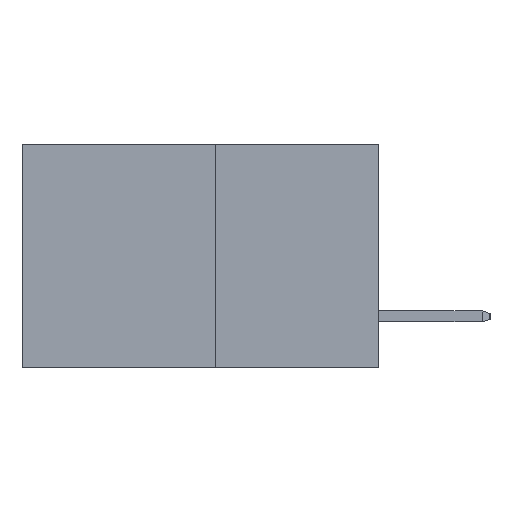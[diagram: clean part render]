
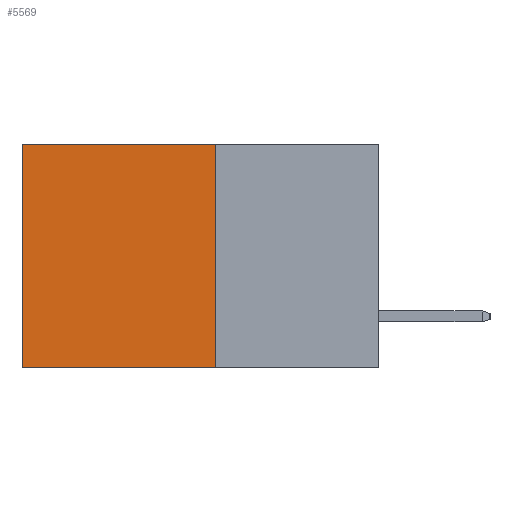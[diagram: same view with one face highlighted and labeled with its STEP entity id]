
A CAD part, left-side view. The second image highlights one B-rep face of the part: STEP entity #5569.
In plain terms, the highlighted planar face has unit normal (-1, 0, 0).
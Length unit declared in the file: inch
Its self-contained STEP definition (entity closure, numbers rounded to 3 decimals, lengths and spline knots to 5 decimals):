
#276 = CARTESIAN_POINT ( 'NONE',  ( 0.277, 0.27, -0.37 ) ) ;
#333 = VERTEX_POINT ( 'NONE', #5721 ) ;
#548 = VERTEX_POINT ( 'NONE', #2251 ) ;
#675 = ORIENTED_EDGE ( 'NONE', *, *, #3470, .F. ) ;
#1112 = DIRECTION ( 'NONE',  ( 1., 0., 0. ) ) ;
#1652 = CARTESIAN_POINT ( 'NONE',  ( 0.277, 0.59, -0.37 ) ) ;
#1995 = DIRECTION ( 'NONE',  ( 0., 1., 0. ) ) ;
#2251 = CARTESIAN_POINT ( 'NONE',  ( 0.277, 0.27, 0. ) ) ;
#2554 = LINE ( 'NONE', #5947, #4457 ) ;
#2792 = CARTESIAN_POINT ( 'NONE',  ( 0.277, 0.27, 0. ) ) ;
#3470 = EDGE_CURVE ( 'NONE', #8673, #333, #2554, .T. ) ;
#3576 = ORIENTED_EDGE ( 'NONE', *, *, #6366, .F. ) ;
#4077 = VECTOR ( 'NONE', #6676, 39.37008 ) ;
#4457 = VECTOR ( 'NONE', #6233, 39.37008 ) ;
#4651 = CARTESIAN_POINT ( 'NONE',  ( 0.277, 0.27, -0.37 ) ) ;
#4746 = AXIS2_PLACEMENT_3D ( 'NONE', #276, #1112, #6191 ) ;
#4806 = PLANE ( 'NONE',  #4746 ) ;
#4910 = EDGE_LOOP ( 'NONE', ( #8149, #675, #3576, #5305 ) ) ;
#4969 = LINE ( 'NONE', #7068, #5188 ) ;
#4987 = LINE ( 'NONE', #2792, #6616 ) ;
#5105 = EDGE_CURVE ( 'NONE', #548, #7210, #4987, .T. ) ;
#5188 = VECTOR ( 'NONE', #6313, 39.37008 ) ;
#5305 = ORIENTED_EDGE ( 'NONE', *, *, #5105, .T. ) ;
#5569 = ADVANCED_FACE ( 'NONE', ( #6395 ), #4806, .F. ) ;
#5721 = CARTESIAN_POINT ( 'NONE',  ( 0.277, 0.59, -0.37 ) ) ;
#5947 = CARTESIAN_POINT ( 'NONE',  ( 0.277, 0.27, -0.37 ) ) ;
#6191 = DIRECTION ( 'NONE',  ( 0., 0., -1. ) ) ;
#6233 = DIRECTION ( 'NONE',  ( 0., 1., 0. ) ) ;
#6313 = DIRECTION ( 'NONE',  ( 0., 0., -1. ) ) ;
#6366 = EDGE_CURVE ( 'NONE', #548, #8673, #4969, .T. ) ;
#6395 = FACE_OUTER_BOUND ( 'NONE', #4910, .T. ) ;
#6616 = VECTOR ( 'NONE', #1995, 39.37008 ) ;
#6676 = DIRECTION ( 'NONE',  ( 0., 0., -1. ) ) ;
#7068 = CARTESIAN_POINT ( 'NONE',  ( 0.277, 0.27, -0.37 ) ) ;
#7210 = VERTEX_POINT ( 'NONE', #7245 ) ;
#7245 = CARTESIAN_POINT ( 'NONE',  ( 0.277, 0.59, 0. ) ) ;
#7330 = EDGE_CURVE ( 'NONE', #7210, #333, #7591, .T. ) ;
#7591 = LINE ( 'NONE', #1652, #4077 ) ;
#8149 = ORIENTED_EDGE ( 'NONE', *, *, #7330, .T. ) ;
#8673 = VERTEX_POINT ( 'NONE', #4651 ) ;
